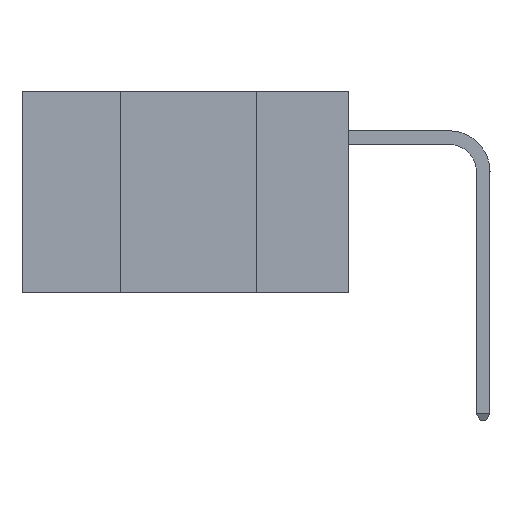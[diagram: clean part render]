
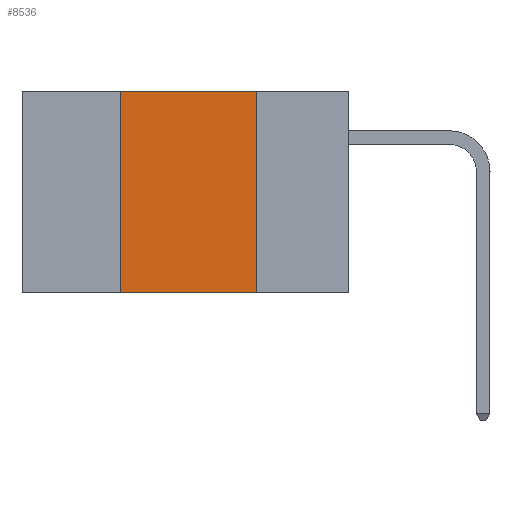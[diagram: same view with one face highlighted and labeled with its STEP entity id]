
A CAD part, left-side view. The second image highlights one B-rep face of the part: STEP entity #8536.
In plain terms, the highlighted planar face has unit normal (-1, 0, 0).
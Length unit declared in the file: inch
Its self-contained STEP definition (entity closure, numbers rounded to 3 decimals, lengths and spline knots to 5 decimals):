
#119 = LINE ( 'NONE', #7531, #12420 ) ;
#521 = CARTESIAN_POINT ( 'NONE',  ( 0., 0.17, -0.37 ) ) ;
#589 = ORIENTED_EDGE ( 'NONE', *, *, #10099, .F. ) ;
#1086 = AXIS2_PLACEMENT_3D ( 'NONE', #12760, #11061, #5257 ) ;
#2635 = LINE ( 'NONE', #6153, #4918 ) ;
#3162 = VERTEX_POINT ( 'NONE', #11511 ) ;
#3387 = CARTESIAN_POINT ( 'NONE',  ( 0., 0.17, 0. ) ) ;
#3500 = ORIENTED_EDGE ( 'NONE', *, *, #7191, .F. ) ;
#4245 = CARTESIAN_POINT ( 'NONE',  ( 0., 0.42, 0. ) ) ;
#4850 = DIRECTION ( 'NONE',  ( 0., -1., 0. ) ) ;
#4918 = VECTOR ( 'NONE', #6859, 39.37008 ) ;
#5257 = DIRECTION ( 'NONE',  ( 0., 0., -1. ) ) ;
#5580 = LINE ( 'NONE', #7726, #11231 ) ;
#5724 = FACE_OUTER_BOUND ( 'NONE', #12967, .T. ) ;
#5891 = CARTESIAN_POINT ( 'NONE',  ( 0., 0.6, -0.37 ) ) ;
#6153 = CARTESIAN_POINT ( 'NONE',  ( 0., 0.42, 0. ) ) ;
#6165 = VERTEX_POINT ( 'NONE', #521 ) ;
#6264 = VECTOR ( 'NONE', #4850, 39.37008 ) ;
#6685 = DIRECTION ( 'NONE',  ( 0., 0., -1. ) ) ;
#6859 = DIRECTION ( 'NONE',  ( 0., 0., 1. ) ) ;
#7191 = EDGE_CURVE ( 'NONE', #8154, #6165, #5580, .T. ) ;
#7531 = CARTESIAN_POINT ( 'NONE',  ( 0., 0.6, 0. ) ) ;
#7726 = CARTESIAN_POINT ( 'NONE',  ( 0., 0.17, 0. ) ) ;
#8154 = VERTEX_POINT ( 'NONE', #3387 ) ;
#8536 = ADVANCED_FACE ( 'NONE', ( #5724 ), #12695, .F. ) ;
#9010 = ORIENTED_EDGE ( 'NONE', *, *, #12882, .T. ) ;
#9686 = DIRECTION ( 'NONE',  ( 0., -1., 0. ) ) ;
#10050 = LINE ( 'NONE', #5891, #6264 ) ;
#10099 = EDGE_CURVE ( 'NONE', #10886, #8154, #119, .T. ) ;
#10886 = VERTEX_POINT ( 'NONE', #4245 ) ;
#11061 = DIRECTION ( 'NONE',  ( 1., 0., 0. ) ) ;
#11231 = VECTOR ( 'NONE', #6685, 39.37008 ) ;
#11511 = CARTESIAN_POINT ( 'NONE',  ( 0., 0.42, -0.37 ) ) ;
#11540 = EDGE_CURVE ( 'NONE', #3162, #10886, #2635, .T. ) ;
#11666 = ORIENTED_EDGE ( 'NONE', *, *, #11540, .F. ) ;
#12420 = VECTOR ( 'NONE', #9686, 39.37008 ) ;
#12695 = PLANE ( 'NONE',  #1086 ) ;
#12760 = CARTESIAN_POINT ( 'NONE',  ( 0., 0.6, 0. ) ) ;
#12882 = EDGE_CURVE ( 'NONE', #3162, #6165, #10050, .T. ) ;
#12967 = EDGE_LOOP ( 'NONE', ( #3500, #589, #11666, #9010 ) ) ;
